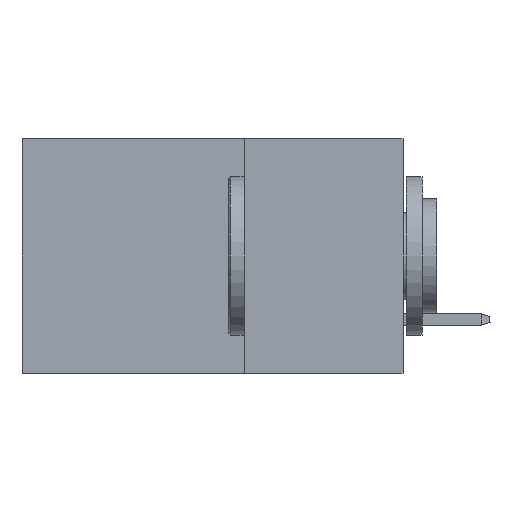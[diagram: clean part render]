
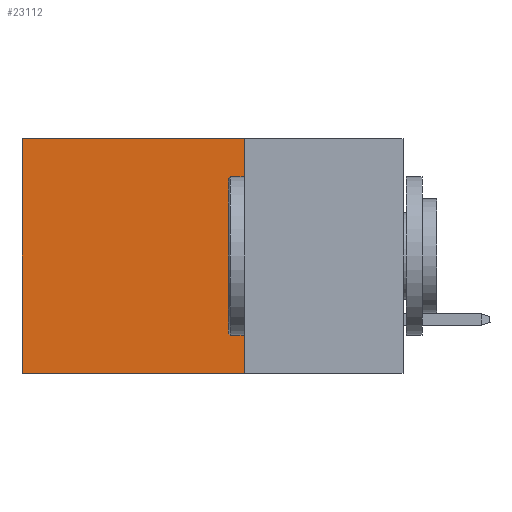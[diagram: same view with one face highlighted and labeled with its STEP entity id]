
A CAD part, left-side view. The second image highlights one B-rep face of the part: STEP entity #23112.
In plain terms, the highlighted planar face has unit normal (-1, 0, 0).
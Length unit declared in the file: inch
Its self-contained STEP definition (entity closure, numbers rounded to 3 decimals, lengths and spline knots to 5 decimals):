
#1888 = CARTESIAN_POINT ( 'NONE',  ( 0.2875, 0.25, -0.37 ) ) ;
#1928 = DIRECTION ( 'NONE',  ( 0., 1., 0. ) ) ;
#3327 = VERTEX_POINT ( 'NONE', #5995 ) ;
#3447 = DIRECTION ( 'NONE',  ( 0., 1., 0. ) ) ;
#3891 = VECTOR ( 'NONE', #1928, 39.37008 ) ;
#4654 = ORIENTED_EDGE ( 'NONE', *, *, #16842, .T. ) ;
#5456 = VERTEX_POINT ( 'NONE', #10887 ) ;
#5814 = VERTEX_POINT ( 'NONE', #19944 ) ;
#5827 = FACE_OUTER_BOUND ( 'NONE', #22915, .T. ) ;
#5995 = CARTESIAN_POINT ( 'NONE',  ( 0.2875, 0.25, 0. ) ) ;
#6287 = DIRECTION ( 'NONE',  ( 0., 0., -1. ) ) ;
#6500 = ORIENTED_EDGE ( 'NONE', *, *, #18014, .F. ) ;
#8479 = VECTOR ( 'NONE', #3447, 39.37008 ) ;
#10127 = AXIS2_PLACEMENT_3D ( 'NONE', #22596, #16946, #20915 ) ;
#10804 = EDGE_CURVE ( 'NONE', #3327, #17630, #20025, .T. ) ;
#10887 = CARTESIAN_POINT ( 'NONE',  ( 0.2875, 0.6, -0.37 ) ) ;
#11614 = LINE ( 'NONE', #14965, #21144 ) ;
#14099 = ORIENTED_EDGE ( 'NONE', *, *, #10804, .T. ) ;
#14562 = VECTOR ( 'NONE', #6287, 39.37008 ) ;
#14862 = CARTESIAN_POINT ( 'NONE',  ( 0.2875, 0.25, 0. ) ) ;
#14965 = CARTESIAN_POINT ( 'NONE',  ( 0.2875, 0.25, 0. ) ) ;
#16842 = EDGE_CURVE ( 'NONE', #17630, #5456, #18735, .T. ) ;
#16946 = DIRECTION ( 'NONE',  ( 1., 0., 0. ) ) ;
#17630 = VERTEX_POINT ( 'NONE', #18803 ) ;
#18014 = EDGE_CURVE ( 'NONE', #5814, #5456, #22238, .T. ) ;
#18735 = LINE ( 'NONE', #22477, #14562 ) ;
#18803 = CARTESIAN_POINT ( 'NONE',  ( 0.2875, 0.6, 0. ) ) ;
#18868 = PLANE ( 'NONE',  #10127 ) ;
#18898 = DIRECTION ( 'NONE',  ( 0., 0., -1. ) ) ;
#19146 = ORIENTED_EDGE ( 'NONE', *, *, #21567, .F. ) ;
#19944 = CARTESIAN_POINT ( 'NONE',  ( 0.2875, 0.25, -0.37 ) ) ;
#20025 = LINE ( 'NONE', #14862, #3891 ) ;
#20915 = DIRECTION ( 'NONE',  ( 0., 0., -1. ) ) ;
#21144 = VECTOR ( 'NONE', #18898, 39.37008 ) ;
#21567 = EDGE_CURVE ( 'NONE', #3327, #5814, #11614, .T. ) ;
#22238 = LINE ( 'NONE', #1888, #8479 ) ;
#22477 = CARTESIAN_POINT ( 'NONE',  ( 0.2875, 0.6, 0. ) ) ;
#22596 = CARTESIAN_POINT ( 'NONE',  ( 0.2875, 0.25, 0. ) ) ;
#22915 = EDGE_LOOP ( 'NONE', ( #4654, #6500, #19146, #14099 ) ) ;
#23112 = ADVANCED_FACE ( 'NONE', ( #5827 ), #18868, .F. ) ;
